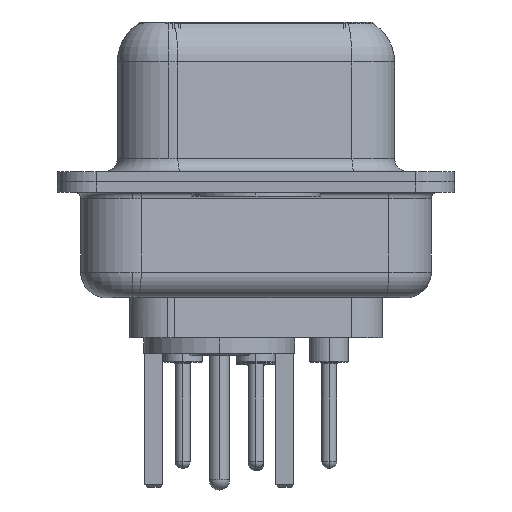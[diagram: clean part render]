
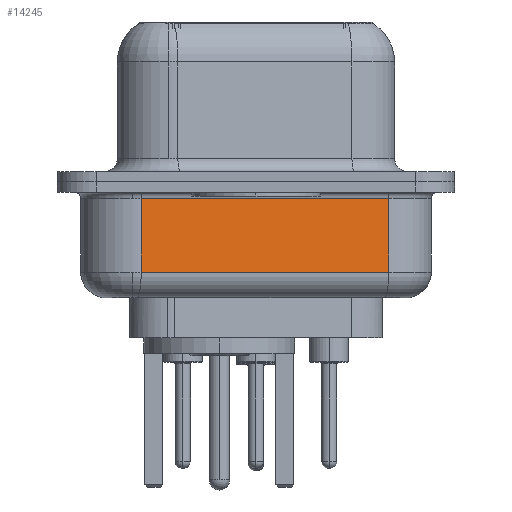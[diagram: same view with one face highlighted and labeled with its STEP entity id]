
A CAD part, left-side view. The second image highlights one B-rep face of the part: STEP entity #14245.
In plain terms, the highlighted planar face has unit normal (-0.985, -0.174, 0).
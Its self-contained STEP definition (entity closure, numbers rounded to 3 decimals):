
#2765 = VECTOR ( 'NONE', #11802, 1000. ) ;
#3502 = LINE ( 'NONE', #15936, #16329 ) ;
#3964 = DIRECTION ( 'NONE',  ( 0., 0., 1. ) ) ;
#4421 = ORIENTED_EDGE ( 'NONE', *, *, #19087, .T. ) ;
#5496 = LINE ( 'NONE', #21837, #2765 ) ;
#5736 = VERTEX_POINT ( 'NONE', #21508 ) ;
#7215 = ORIENTED_EDGE ( 'NONE', *, *, #15020, .T. ) ;
#7450 = ORIENTED_EDGE ( 'NONE', *, *, #21120, .F. ) ;
#9857 = AXIS2_PLACEMENT_3D ( 'NONE', #32144, #29473, #17252 ) ;
#11802 = DIRECTION ( 'NONE',  ( 0., 0., 1. ) ) ;
#14095 = VECTOR ( 'NONE', #3964, 1000. ) ;
#14245 = ADVANCED_FACE ( 'NONE', ( #19445 ), #24474, .F. ) ;
#15020 = EDGE_CURVE ( 'NONE', #26483, #15517, #3502, .T. ) ;
#15517 = VERTEX_POINT ( 'NONE', #29772 ) ;
#15936 = CARTESIAN_POINT ( 'NONE',  ( 2.93, 4.453, -0.65 ) ) ;
#16329 = VECTOR ( 'NONE', #30980, 1000. ) ;
#17252 = DIRECTION ( 'NONE',  ( -0.174, 0.985, 0. ) ) ;
#17345 = LINE ( 'NONE', #29035, #20025 ) ;
#19087 = EDGE_CURVE ( 'NONE', #5736, #20289, #17345, .T. ) ;
#19445 = FACE_OUTER_BOUND ( 'NONE', #20864, .T. ) ;
#20025 = VECTOR ( 'NONE', #31525, 1000. ) ;
#20289 = VERTEX_POINT ( 'NONE', #27296 ) ;
#20864 = EDGE_LOOP ( 'NONE', ( #7450, #4421, #23514, #7215 ) ) ;
#21120 = EDGE_CURVE ( 'NONE', #5736, #15517, #31543, .T. ) ;
#21508 = CARTESIAN_POINT ( 'NONE',  ( 2.93, 4.453, -3.5 ) ) ;
#21837 = CARTESIAN_POINT ( 'NONE',  ( 4.623, -5.147, -4.5 ) ) ;
#22510 = CARTESIAN_POINT ( 'NONE',  ( 4.623, -5.147, -0.65 ) ) ;
#23514 = ORIENTED_EDGE ( 'NONE', *, *, #23823, .T. ) ;
#23823 = EDGE_CURVE ( 'NONE', #20289, #26483, #5496, .T. ) ;
#23874 = CARTESIAN_POINT ( 'NONE',  ( 2.93, 4.453, -4.5 ) ) ;
#24474 = PLANE ( 'NONE',  #9857 ) ;
#26483 = VERTEX_POINT ( 'NONE', #22510 ) ;
#27296 = CARTESIAN_POINT ( 'NONE',  ( 4.623, -5.147, -3.5 ) ) ;
#29035 = CARTESIAN_POINT ( 'NONE',  ( 2.93, 4.453, -3.5 ) ) ;
#29473 = DIRECTION ( 'NONE',  ( 0.985, 0.174, 0. ) ) ;
#29772 = CARTESIAN_POINT ( 'NONE',  ( 2.93, 4.453, -0.65 ) ) ;
#30980 = DIRECTION ( 'NONE',  ( -0.174, 0.985, 0. ) ) ;
#31525 = DIRECTION ( 'NONE',  ( 0.174, -0.985, 0. ) ) ;
#31543 = LINE ( 'NONE', #23874, #14095 ) ;
#32144 = CARTESIAN_POINT ( 'NONE',  ( 2.93, 4.453, -4.5 ) ) ;
